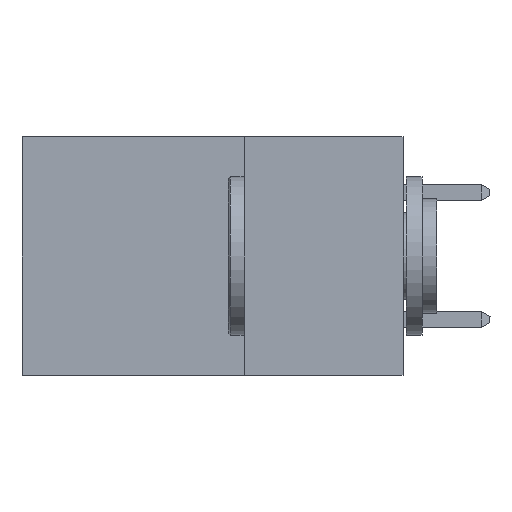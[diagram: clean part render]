
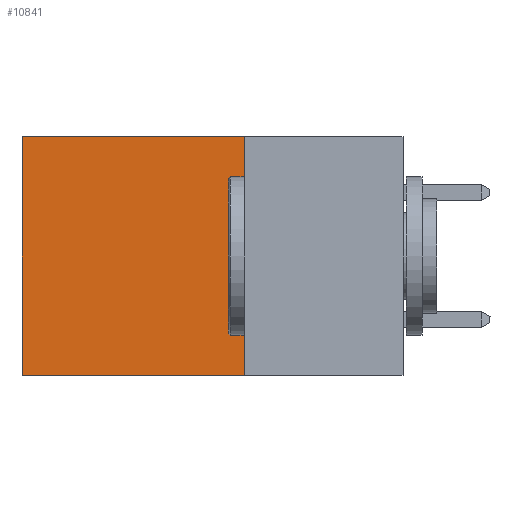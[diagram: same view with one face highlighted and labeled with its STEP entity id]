
A CAD part, left-side view. The second image highlights one B-rep face of the part: STEP entity #10841.
In plain terms, the highlighted planar face has unit normal (-1, 0, 0).
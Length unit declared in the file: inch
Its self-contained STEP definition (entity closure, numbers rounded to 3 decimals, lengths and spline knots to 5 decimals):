
#185 = CARTESIAN_POINT ( 'NONE',  ( 0.2875, 0.25, -0.375 ) ) ;
#849 = EDGE_LOOP ( 'NONE', ( #9305, #14536, #15666, #17981 ) ) ;
#1026 = CARTESIAN_POINT ( 'NONE',  ( 0.2875, 0.6, -0.375 ) ) ;
#1702 = CARTESIAN_POINT ( 'NONE',  ( 0.2875, 0.25, -0.375 ) ) ;
#2023 = EDGE_CURVE ( 'NONE', #8193, #8845, #19017, .T. ) ;
#2487 = VECTOR ( 'NONE', #12971, 39.37008 ) ;
#2542 = EDGE_CURVE ( 'NONE', #12637, #2911, #5994, .T. ) ;
#2911 = VERTEX_POINT ( 'NONE', #4936 ) ;
#4936 = CARTESIAN_POINT ( 'NONE',  ( 0.2875, 0.6, -0.375 ) ) ;
#4960 = PLANE ( 'NONE',  #15166 ) ;
#5315 = CARTESIAN_POINT ( 'NONE',  ( 0.2875, 0.25, -0.375 ) ) ;
#5994 = LINE ( 'NONE', #1026, #2487 ) ;
#6841 = LINE ( 'NONE', #17100, #16522 ) ;
#7417 = EDGE_CURVE ( 'NONE', #8193, #12637, #10123, .T. ) ;
#7779 = DIRECTION ( 'NONE',  ( 1., 0., 0. ) ) ;
#8193 = VERTEX_POINT ( 'NONE', #17144 ) ;
#8845 = VERTEX_POINT ( 'NONE', #1702 ) ;
#9305 = ORIENTED_EDGE ( 'NONE', *, *, #2542, .T. ) ;
#9438 = DIRECTION ( 'NONE',  ( 0., 1., 0. ) ) ;
#9813 = VECTOR ( 'NONE', #12884, 39.37008 ) ;
#10123 = LINE ( 'NONE', #13713, #10599 ) ;
#10599 = VECTOR ( 'NONE', #9438, 39.37008 ) ;
#10706 = DIRECTION ( 'NONE',  ( 0., 0., -1. ) ) ;
#10841 = ADVANCED_FACE ( 'NONE', ( #18583 ), #4960, .F. ) ;
#12637 = VERTEX_POINT ( 'NONE', #13538 ) ;
#12884 = DIRECTION ( 'NONE',  ( 0., 0., -1. ) ) ;
#12971 = DIRECTION ( 'NONE',  ( 0., 0., -1. ) ) ;
#13538 = CARTESIAN_POINT ( 'NONE',  ( 0.2875, 0.6, 0. ) ) ;
#13713 = CARTESIAN_POINT ( 'NONE',  ( 0.2875, 0.25, 0. ) ) ;
#14059 = DIRECTION ( 'NONE',  ( 0., 1., 0. ) ) ;
#14536 = ORIENTED_EDGE ( 'NONE', *, *, #15589, .F. ) ;
#15166 = AXIS2_PLACEMENT_3D ( 'NONE', #185, #7779, #10706 ) ;
#15589 = EDGE_CURVE ( 'NONE', #8845, #2911, #6841, .T. ) ;
#15666 = ORIENTED_EDGE ( 'NONE', *, *, #2023, .F. ) ;
#16522 = VECTOR ( 'NONE', #14059, 39.37008 ) ;
#17100 = CARTESIAN_POINT ( 'NONE',  ( 0.2875, 0.25, -0.375 ) ) ;
#17144 = CARTESIAN_POINT ( 'NONE',  ( 0.2875, 0.25, 0. ) ) ;
#17981 = ORIENTED_EDGE ( 'NONE', *, *, #7417, .T. ) ;
#18583 = FACE_OUTER_BOUND ( 'NONE', #849, .T. ) ;
#19017 = LINE ( 'NONE', #5315, #9813 ) ;
